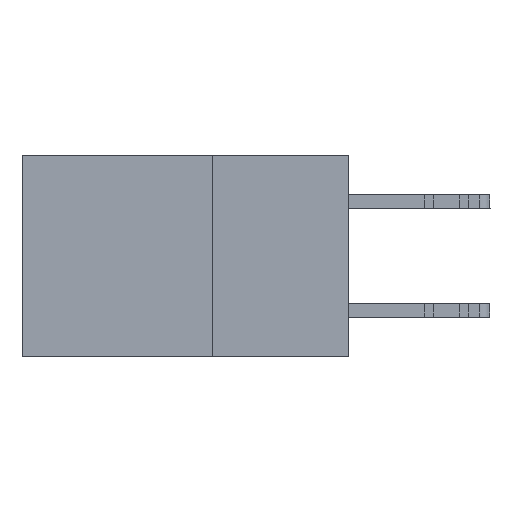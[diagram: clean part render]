
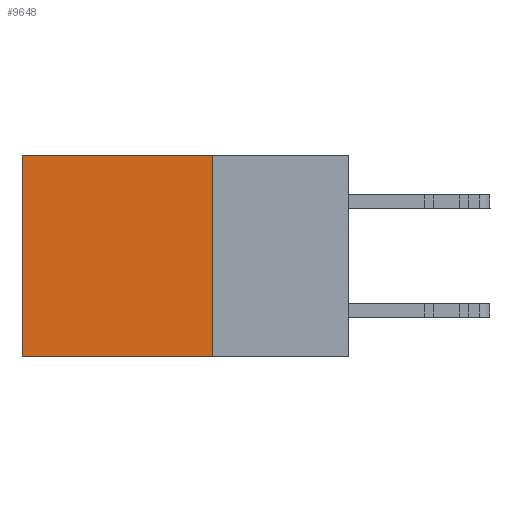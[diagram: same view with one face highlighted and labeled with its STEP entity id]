
A CAD part, left-side view. The second image highlights one B-rep face of the part: STEP entity #9648.
In plain terms, the highlighted planar face has unit normal (-1, 0, 0).
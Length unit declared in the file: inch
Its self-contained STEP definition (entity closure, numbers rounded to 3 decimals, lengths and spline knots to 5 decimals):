
#20 = CARTESIAN_POINT ( 'NONE',  ( 0.2615, 0.25, -0.37 ) ) ;
#81 = VECTOR ( 'NONE', #23307, 39.37008 ) ;
#2119 = EDGE_LOOP ( 'NONE', ( #2666, #24810, #16620, #24297 ) ) ;
#2618 = VERTEX_POINT ( 'NONE', #11866 ) ;
#2666 = ORIENTED_EDGE ( 'NONE', *, *, #3434, .T. ) ;
#3075 = CARTESIAN_POINT ( 'NONE',  ( 0.2615, 0.6, -0.37 ) ) ;
#3434 = EDGE_CURVE ( 'NONE', #8719, #9442, #23219, .T. ) ;
#5687 = CARTESIAN_POINT ( 'NONE',  ( 0.2615, 0.25, -0.37 ) ) ;
#5900 = CARTESIAN_POINT ( 'NONE',  ( 0.2615, 0.25, -0.37 ) ) ;
#8521 = CARTESIAN_POINT ( 'NONE',  ( 0.2615, 0.25, -0.37 ) ) ;
#8719 = VERTEX_POINT ( 'NONE', #17433 ) ;
#9080 = CARTESIAN_POINT ( 'NONE',  ( 0.2615, 0.6, -0.37 ) ) ;
#9287 = LINE ( 'NONE', #11124, #81 ) ;
#9442 = VERTEX_POINT ( 'NONE', #3075 ) ;
#9648 = ADVANCED_FACE ( 'NONE', ( #19537 ), #23288, .F. ) ;
#9650 = DIRECTION ( 'NONE',  ( 0., 0., -1. ) ) ;
#11124 = CARTESIAN_POINT ( 'NONE',  ( 0.2615, 0.25, 0. ) ) ;
#11407 = DIRECTION ( 'NONE',  ( 0., 0., -1. ) ) ;
#11866 = CARTESIAN_POINT ( 'NONE',  ( 0.2615, 0.25, 0. ) ) ;
#12354 = AXIS2_PLACEMENT_3D ( 'NONE', #5900, #23808, #9650 ) ;
#12431 = EDGE_CURVE ( 'NONE', #23663, #9442, #15552, .T. ) ;
#12549 = DIRECTION ( 'NONE',  ( 0., 0., -1. ) ) ;
#14017 = EDGE_CURVE ( 'NONE', #2618, #8719, #9287, .T. ) ;
#15110 = VECTOR ( 'NONE', #11407, 39.37008 ) ;
#15552 = LINE ( 'NONE', #5687, #18278 ) ;
#16544 = EDGE_CURVE ( 'NONE', #2618, #23663, #22409, .T. ) ;
#16620 = ORIENTED_EDGE ( 'NONE', *, *, #16544, .F. ) ;
#17433 = CARTESIAN_POINT ( 'NONE',  ( 0.2615, 0.6, 0. ) ) ;
#18278 = VECTOR ( 'NONE', #24330, 39.37008 ) ;
#19537 = FACE_OUTER_BOUND ( 'NONE', #2119, .T. ) ;
#22409 = LINE ( 'NONE', #8521, #23964 ) ;
#23219 = LINE ( 'NONE', #9080, #15110 ) ;
#23288 = PLANE ( 'NONE',  #12354 ) ;
#23307 = DIRECTION ( 'NONE',  ( 0., 1., 0. ) ) ;
#23663 = VERTEX_POINT ( 'NONE', #20 ) ;
#23808 = DIRECTION ( 'NONE',  ( 1., 0., 0. ) ) ;
#23964 = VECTOR ( 'NONE', #12549, 39.37008 ) ;
#24297 = ORIENTED_EDGE ( 'NONE', *, *, #14017, .T. ) ;
#24330 = DIRECTION ( 'NONE',  ( 0., 1., 0. ) ) ;
#24810 = ORIENTED_EDGE ( 'NONE', *, *, #12431, .F. ) ;
